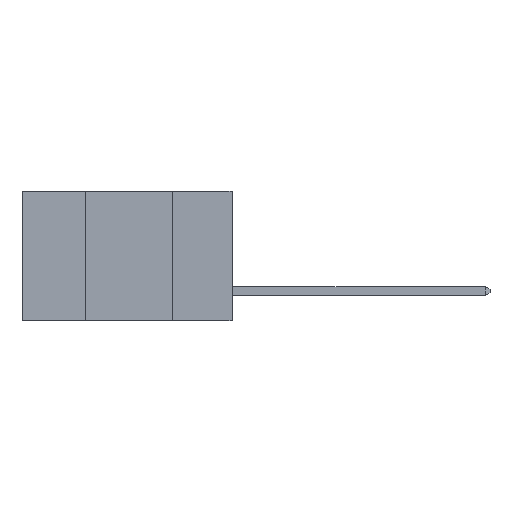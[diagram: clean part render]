
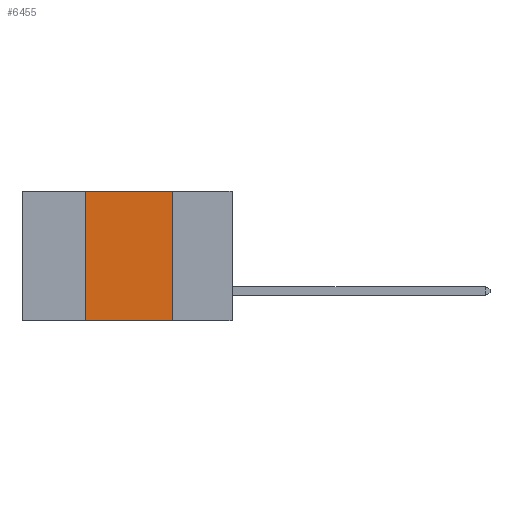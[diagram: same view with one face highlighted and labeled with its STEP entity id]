
A CAD part, left-side view. The second image highlights one B-rep face of the part: STEP entity #6455.
In plain terms, the highlighted planar face has unit normal (-1, 0, 0).
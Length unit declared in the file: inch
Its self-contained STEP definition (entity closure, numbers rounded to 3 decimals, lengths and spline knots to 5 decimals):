
#750 = VECTOR ( 'NONE', #7580, 39.37008 ) ;
#1541 = VERTEX_POINT ( 'NONE', #17536 ) ;
#1631 = LINE ( 'NONE', #16520, #13753 ) ;
#1646 = DIRECTION ( 'NONE',  ( 0., 0., -1. ) ) ;
#1967 = EDGE_CURVE ( 'NONE', #10797, #15613, #1631, .T. ) ;
#2882 = VECTOR ( 'NONE', #1646, 39.37008 ) ;
#2985 = LINE ( 'NONE', #17907, #3498 ) ;
#3457 = CARTESIAN_POINT ( 'NONE',  ( 0., 0.17, 0. ) ) ;
#3498 = VECTOR ( 'NONE', #9099, 39.37008 ) ;
#5123 = CARTESIAN_POINT ( 'NONE',  ( 0., 0.42, -0.37 ) ) ;
#5251 = CARTESIAN_POINT ( 'NONE',  ( 0., 0.42, 0. ) ) ;
#5357 = EDGE_CURVE ( 'NONE', #6974, #10797, #11994, .T. ) ;
#6455 = ADVANCED_FACE ( 'NONE', ( #18063 ), #16228, .F. ) ;
#6974 = VERTEX_POINT ( 'NONE', #5123 ) ;
#7407 = ORIENTED_EDGE ( 'NONE', *, *, #19691, .F. ) ;
#7522 = EDGE_CURVE ( 'NONE', #6974, #1541, #2985, .T. ) ;
#7580 = DIRECTION ( 'NONE',  ( 0., 0., 1. ) ) ;
#7632 = ORIENTED_EDGE ( 'NONE', *, *, #1967, .F. ) ;
#7654 = ORIENTED_EDGE ( 'NONE', *, *, #5357, .F. ) ;
#8018 = ORIENTED_EDGE ( 'NONE', *, *, #7522, .T. ) ;
#8233 = LINE ( 'NONE', #11245, #2882 ) ;
#8823 = DIRECTION ( 'NONE',  ( 0., 0., -1. ) ) ;
#9099 = DIRECTION ( 'NONE',  ( 0., -1., 0. ) ) ;
#10797 = VERTEX_POINT ( 'NONE', #5251 ) ;
#11245 = CARTESIAN_POINT ( 'NONE',  ( 0., 0.17, 0. ) ) ;
#11826 = CARTESIAN_POINT ( 'NONE',  ( 0., 0.6, 0. ) ) ;
#11994 = LINE ( 'NONE', #16518, #750 ) ;
#13753 = VECTOR ( 'NONE', #14043, 39.37008 ) ;
#14043 = DIRECTION ( 'NONE',  ( 0., -1., 0. ) ) ;
#15613 = VERTEX_POINT ( 'NONE', #3457 ) ;
#16228 = PLANE ( 'NONE',  #18403 ) ;
#16518 = CARTESIAN_POINT ( 'NONE',  ( 0., 0.42, 0. ) ) ;
#16520 = CARTESIAN_POINT ( 'NONE',  ( 0., 0.6, 0. ) ) ;
#17536 = CARTESIAN_POINT ( 'NONE',  ( 0., 0.17, -0.37 ) ) ;
#17674 = DIRECTION ( 'NONE',  ( 1., 0., 0. ) ) ;
#17693 = EDGE_LOOP ( 'NONE', ( #7407, #7632, #7654, #8018 ) ) ;
#17907 = CARTESIAN_POINT ( 'NONE',  ( 0., 0.6, -0.37 ) ) ;
#18063 = FACE_OUTER_BOUND ( 'NONE', #17693, .T. ) ;
#18403 = AXIS2_PLACEMENT_3D ( 'NONE', #11826, #17674, #8823 ) ;
#19691 = EDGE_CURVE ( 'NONE', #15613, #1541, #8233, .T. ) ;
